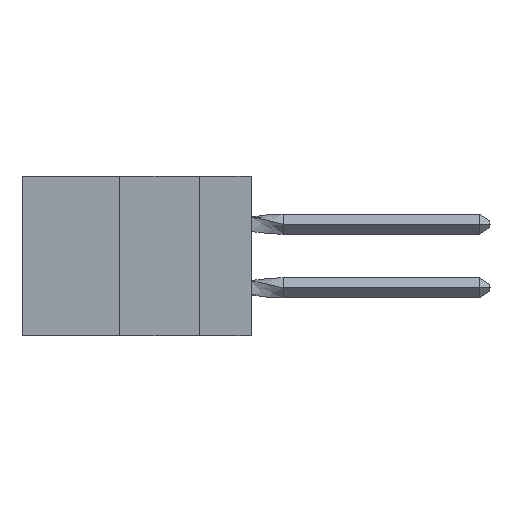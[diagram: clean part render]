
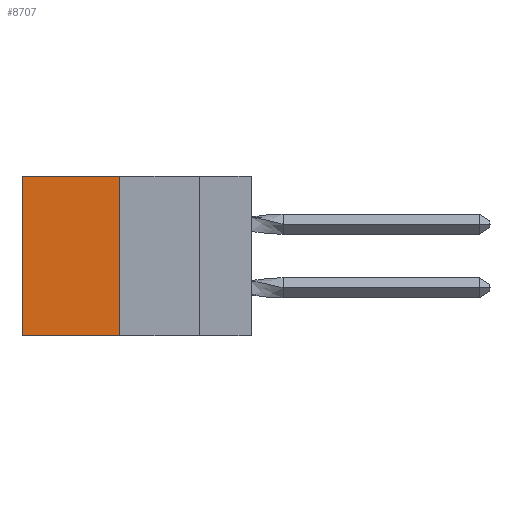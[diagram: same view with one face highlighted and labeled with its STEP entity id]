
A CAD part, left-side view. The second image highlights one B-rep face of the part: STEP entity #8707.
In plain terms, the highlighted planar face has unit normal (-1, 0, 0).
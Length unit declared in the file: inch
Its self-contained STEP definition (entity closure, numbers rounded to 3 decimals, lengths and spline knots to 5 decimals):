
#1049 = CARTESIAN_POINT ( 'NONE',  ( 0.305, 0.72, 0. ) ) ;
#2380 = ORIENTED_EDGE ( 'NONE', *, *, #19982, .F. ) ;
#3206 = LINE ( 'NONE', #8742, #8194 ) ;
#3793 = EDGE_CURVE ( 'NONE', #18147, #9833, #12047, .T. ) ;
#4773 = VERTEX_POINT ( 'NONE', #1049 ) ;
#4889 = DIRECTION ( 'NONE',  ( 0., 0., -1. ) ) ;
#7744 = CARTESIAN_POINT ( 'NONE',  ( 0.305, 0.72, -0.5 ) ) ;
#7858 = CARTESIAN_POINT ( 'NONE',  ( 0.305, 0.413, -0.5 ) ) ;
#8194 = VECTOR ( 'NONE', #19935, 39.37008 ) ;
#8441 = VECTOR ( 'NONE', #23168, 39.37008 ) ;
#8707 = ADVANCED_FACE ( 'NONE', ( #10727 ), #18360, .F. ) ;
#8742 = CARTESIAN_POINT ( 'NONE',  ( 0.305, 0.72, -0.5 ) ) ;
#9833 = VERTEX_POINT ( 'NONE', #7744 ) ;
#10727 = FACE_OUTER_BOUND ( 'NONE', #12724, .T. ) ;
#12047 = LINE ( 'NONE', #22911, #13517 ) ;
#12230 = VERTEX_POINT ( 'NONE', #18793 ) ;
#12469 = DIRECTION ( 'NONE',  ( 0., 0., -1. ) ) ;
#12724 = EDGE_LOOP ( 'NONE', ( #22613, #15864, #2380, #20382 ) ) ;
#13517 = VECTOR ( 'NONE', #19200, 39.37008 ) ;
#14364 = AXIS2_PLACEMENT_3D ( 'NONE', #21966, #21805, #12469 ) ;
#15527 = LINE ( 'NONE', #21196, #17317 ) ;
#15864 = ORIENTED_EDGE ( 'NONE', *, *, #3793, .F. ) ;
#16268 = EDGE_CURVE ( 'NONE', #12230, #4773, #16963, .T. ) ;
#16963 = LINE ( 'NONE', #17518, #8441 ) ;
#17317 = VECTOR ( 'NONE', #4889, 39.37008 ) ;
#17518 = CARTESIAN_POINT ( 'NONE',  ( 0.305, 0.413, 0. ) ) ;
#18147 = VERTEX_POINT ( 'NONE', #7858 ) ;
#18360 = PLANE ( 'NONE',  #14364 ) ;
#18793 = CARTESIAN_POINT ( 'NONE',  ( 0.305, 0.413, 0. ) ) ;
#19200 = DIRECTION ( 'NONE',  ( 0., 1., 0. ) ) ;
#19771 = EDGE_CURVE ( 'NONE', #4773, #9833, #3206, .T. ) ;
#19935 = DIRECTION ( 'NONE',  ( 0., 0., -1. ) ) ;
#19982 = EDGE_CURVE ( 'NONE', #12230, #18147, #15527, .T. ) ;
#20382 = ORIENTED_EDGE ( 'NONE', *, *, #16268, .T. ) ;
#21196 = CARTESIAN_POINT ( 'NONE',  ( 0.305, 0.413, -0.5 ) ) ;
#21805 = DIRECTION ( 'NONE',  ( 1., 0., 0. ) ) ;
#21966 = CARTESIAN_POINT ( 'NONE',  ( 0.305, 0.413, -0.5 ) ) ;
#22613 = ORIENTED_EDGE ( 'NONE', *, *, #19771, .T. ) ;
#22911 = CARTESIAN_POINT ( 'NONE',  ( 0.305, 0.413, -0.5 ) ) ;
#23168 = DIRECTION ( 'NONE',  ( 0., 1., 0. ) ) ;
